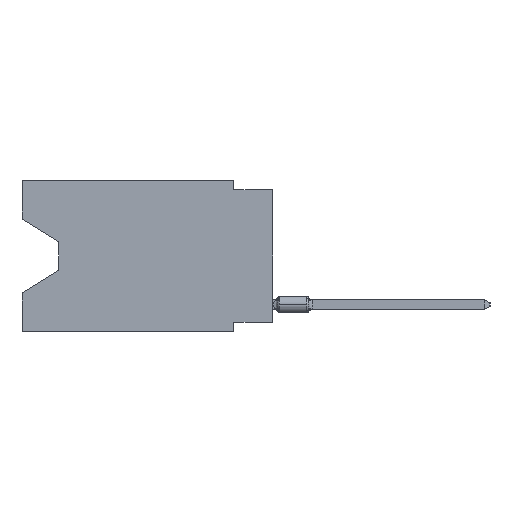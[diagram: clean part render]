
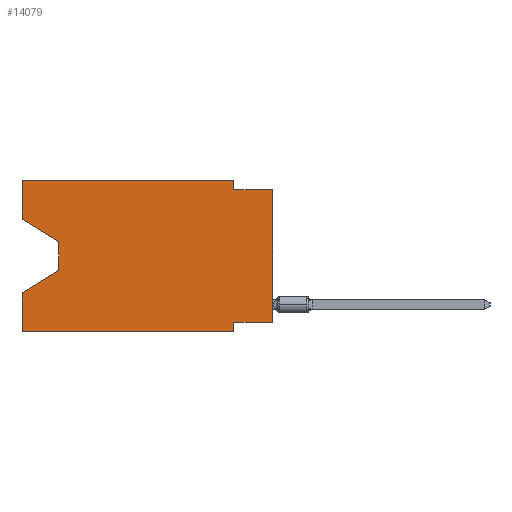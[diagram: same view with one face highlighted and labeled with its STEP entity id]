
A CAD part, left-side view. The second image highlights one B-rep face of the part: STEP entity #14079.
In plain terms, the highlighted planar face has unit normal (-1, 0, 0).
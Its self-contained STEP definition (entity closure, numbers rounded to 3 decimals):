
#328 = LINE ( 'NONE', #13141, #53529 ) ;
#498 = VERTEX_POINT ( 'NONE', #5174 ) ;
#755 = DIRECTION ( 'NONE',  ( 0., 0., -1. ) ) ;
#1283 = EDGE_CURVE ( 'NONE', #43343, #44534, #22998, .T. ) ;
#1844 = CARTESIAN_POINT ( 'NONE',  ( 0., 0., -0.635 ) ) ;
#2564 = CARTESIAN_POINT ( 'NONE',  ( 0., 16.383, -2.546 ) ) ;
#4125 = EDGE_LOOP ( 'NONE', ( #4890, #27579, #42193, #14277, #19822, #36843, #50276, #24381, #23565, #43299, #37609, #25254 ) ) ;
#4242 = LINE ( 'NONE', #50309, #13818 ) ;
#4783 = EDGE_CURVE ( 'NONE', #14409, #48817, #17700, .T. ) ;
#4890 = ORIENTED_EDGE ( 'NONE', *, *, #32805, .T. ) ;
#5021 = DIRECTION ( 'NONE',  ( 0., 0., -1. ) ) ;
#5174 = CARTESIAN_POINT ( 'NONE',  ( 0., 2.54, -9.271 ) ) ;
#7124 = CARTESIAN_POINT ( 'NONE',  ( 0., 13.97, -5.893 ) ) ;
#8241 = VERTEX_POINT ( 'NONE', #36587 ) ;
#8855 = CARTESIAN_POINT ( 'NONE',  ( 0., 2.54, -9.906 ) ) ;
#9750 = VECTOR ( 'NONE', #5021, 1000. ) ;
#10159 = CARTESIAN_POINT ( 'NONE',  ( 0., 16.383, 0. ) ) ;
#11383 = DIRECTION ( 'NONE',  ( 0., -1., 0. ) ) ;
#11391 = LINE ( 'NONE', #44671, #20614 ) ;
#11428 = CARTESIAN_POINT ( 'NONE',  ( 0., 13.97, -4.013 ) ) ;
#11987 = VECTOR ( 'NONE', #755, 1000. ) ;
#12860 = VECTOR ( 'NONE', #43983, 1000. ) ;
#13141 = CARTESIAN_POINT ( 'NONE',  ( 0., 16.383, 0. ) ) ;
#13259 = DIRECTION ( 'NONE',  ( 0., 0., -1. ) ) ;
#13790 = EDGE_CURVE ( 'NONE', #498, #8241, #25528, .T. ) ;
#13818 = VECTOR ( 'NONE', #50844, 1000. ) ;
#14079 = ADVANCED_FACE ( 'NONE', ( #50607 ), #50072, .F. ) ;
#14277 = ORIENTED_EDGE ( 'NONE', *, *, #19784, .F. ) ;
#14409 = VERTEX_POINT ( 'NONE', #31286 ) ;
#15039 = CARTESIAN_POINT ( 'NONE',  ( 0., 0., -9.271 ) ) ;
#16865 = DIRECTION ( 'NONE',  ( 1., 0., 0. ) ) ;
#16868 = CARTESIAN_POINT ( 'NONE',  ( 0., 13.97, -5.893 ) ) ;
#16903 = LINE ( 'NONE', #33797, #11987 ) ;
#17426 = DIRECTION ( 'NONE',  ( 0., 0., -1. ) ) ;
#17700 = LINE ( 'NONE', #43594, #47139 ) ;
#18506 = EDGE_CURVE ( 'NONE', #48817, #29520, #11391, .T. ) ;
#19780 = LINE ( 'NONE', #2564, #47813 ) ;
#19784 = EDGE_CURVE ( 'NONE', #53088, #44534, #46802, .T. ) ;
#19822 = ORIENTED_EDGE ( 'NONE', *, *, #51390, .T. ) ;
#20318 = DIRECTION ( 'NONE',  ( 0., -0.855, -0.519 ) ) ;
#20533 = CARTESIAN_POINT ( 'NONE',  ( 0., 16.383, -2.546 ) ) ;
#20614 = VECTOR ( 'NONE', #53351, 1000. ) ;
#21118 = AXIS2_PLACEMENT_3D ( 'NONE', #34021, #16865, #13259 ) ;
#21626 = VECTOR ( 'NONE', #31691, 1000. ) ;
#22998 = LINE ( 'NONE', #7124, #12860 ) ;
#23427 = LINE ( 'NONE', #48728, #25617 ) ;
#23565 = ORIENTED_EDGE ( 'NONE', *, *, #18506, .F. ) ;
#23683 = CARTESIAN_POINT ( 'NONE',  ( 0., 2.54, -0.635 ) ) ;
#23894 = CARTESIAN_POINT ( 'NONE',  ( 0., 16.383, 0. ) ) ;
#24381 = ORIENTED_EDGE ( 'NONE', *, *, #32561, .T. ) ;
#25254 = ORIENTED_EDGE ( 'NONE', *, *, #27059, .F. ) ;
#25528 = LINE ( 'NONE', #8855, #9750 ) ;
#25617 = VECTOR ( 'NONE', #11383, 1000. ) ;
#27059 = EDGE_CURVE ( 'NONE', #38118, #51029, #328, .T. ) ;
#27579 = ORIENTED_EDGE ( 'NONE', *, *, #48469, .T. ) ;
#28660 = EDGE_CURVE ( 'NONE', #50604, #498, #52893, .T. ) ;
#29224 = CARTESIAN_POINT ( 'NONE',  ( 0., 16.383, -7.36 ) ) ;
#29520 = VERTEX_POINT ( 'NONE', #1844 ) ;
#31286 = CARTESIAN_POINT ( 'NONE',  ( 0., 2.54, 0. ) ) ;
#31691 = DIRECTION ( 'NONE',  ( 0., 1., 0. ) ) ;
#32561 = EDGE_CURVE ( 'NONE', #50604, #29520, #4242, .T. ) ;
#32799 = EDGE_CURVE ( 'NONE', #51029, #14409, #52481, .T. ) ;
#32805 = EDGE_CURVE ( 'NONE', #38118, #45495, #19780, .T. ) ;
#33797 = CARTESIAN_POINT ( 'NONE',  ( 0., 13.97, -4.013 ) ) ;
#34021 = CARTESIAN_POINT ( 'NONE',  ( 0., 16.383, 0. ) ) ;
#36587 = CARTESIAN_POINT ( 'NONE',  ( 0., 2.54, -9.906 ) ) ;
#36843 = ORIENTED_EDGE ( 'NONE', *, *, #13790, .F. ) ;
#37310 = CARTESIAN_POINT ( 'NONE',  ( 0., 16.383, 0. ) ) ;
#37609 = ORIENTED_EDGE ( 'NONE', *, *, #32799, .F. ) ;
#38118 = VERTEX_POINT ( 'NONE', #20533 ) ;
#40241 = DIRECTION ( 'NONE',  ( 0., -1., 0. ) ) ;
#42193 = ORIENTED_EDGE ( 'NONE', *, *, #1283, .T. ) ;
#43299 = ORIENTED_EDGE ( 'NONE', *, *, #4783, .F. ) ;
#43343 = VERTEX_POINT ( 'NONE', #16868 ) ;
#43473 = VECTOR ( 'NONE', #40241, 1000. ) ;
#43590 = CARTESIAN_POINT ( 'NONE',  ( 0., 16.383, -9.906 ) ) ;
#43594 = CARTESIAN_POINT ( 'NONE',  ( 0., 2.54, 0. ) ) ;
#43983 = DIRECTION ( 'NONE',  ( 0., 0.855, -0.519 ) ) ;
#44062 = CARTESIAN_POINT ( 'NONE',  ( 0., 0., -9.271 ) ) ;
#44534 = VERTEX_POINT ( 'NONE', #29224 ) ;
#44671 = CARTESIAN_POINT ( 'NONE',  ( 0., 0., -0.635 ) ) ;
#45495 = VERTEX_POINT ( 'NONE', #11428 ) ;
#45999 = DIRECTION ( 'NONE',  ( 0., 0., 1. ) ) ;
#46802 = LINE ( 'NONE', #37310, #48913 ) ;
#47139 = VECTOR ( 'NONE', #17426, 1000. ) ;
#47813 = VECTOR ( 'NONE', #20318, 1000. ) ;
#48469 = EDGE_CURVE ( 'NONE', #45495, #43343, #16903, .T. ) ;
#48728 = CARTESIAN_POINT ( 'NONE',  ( 0., 16.383, -9.906 ) ) ;
#48817 = VERTEX_POINT ( 'NONE', #23683 ) ;
#48913 = VECTOR ( 'NONE', #45999, 1000. ) ;
#50072 = PLANE ( 'NONE',  #21118 ) ;
#50276 = ORIENTED_EDGE ( 'NONE', *, *, #28660, .F. ) ;
#50309 = CARTESIAN_POINT ( 'NONE',  ( 0., 0., 0. ) ) ;
#50604 = VERTEX_POINT ( 'NONE', #44062 ) ;
#50607 = FACE_OUTER_BOUND ( 'NONE', #4125, .T. ) ;
#50754 = DIRECTION ( 'NONE',  ( 0., 0., 1. ) ) ;
#50844 = DIRECTION ( 'NONE',  ( 0., 0., 1. ) ) ;
#51029 = VERTEX_POINT ( 'NONE', #10159 ) ;
#51390 = EDGE_CURVE ( 'NONE', #53088, #8241, #23427, .T. ) ;
#52481 = LINE ( 'NONE', #23894, #43473 ) ;
#52893 = LINE ( 'NONE', #15039, #21626 ) ;
#53088 = VERTEX_POINT ( 'NONE', #43590 ) ;
#53351 = DIRECTION ( 'NONE',  ( 0., -1., 0. ) ) ;
#53529 = VECTOR ( 'NONE', #50754, 1000. ) ;
